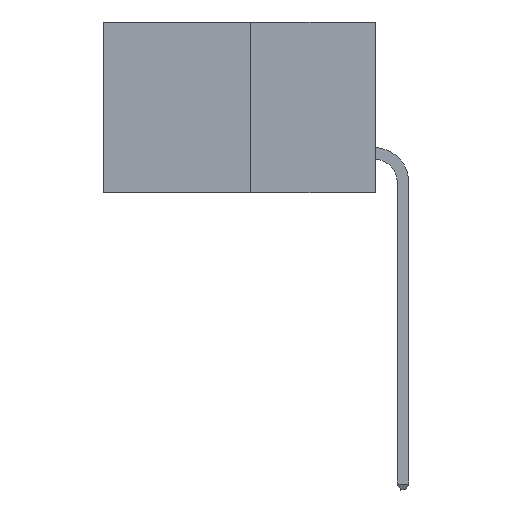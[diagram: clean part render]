
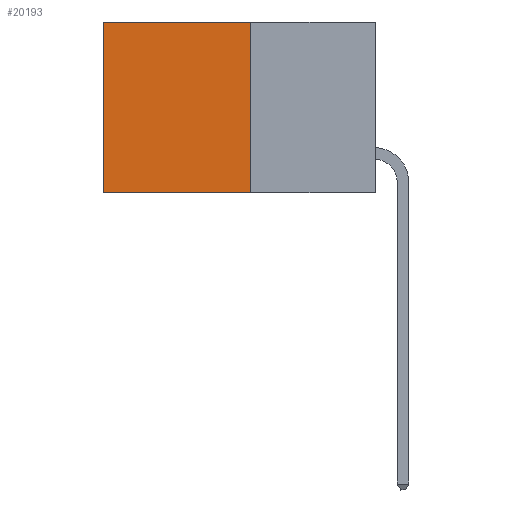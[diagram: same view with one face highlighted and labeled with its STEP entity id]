
A CAD part, left-side view. The second image highlights one B-rep face of the part: STEP entity #20193.
In plain terms, the highlighted planar face has unit normal (-1, 0, 0).
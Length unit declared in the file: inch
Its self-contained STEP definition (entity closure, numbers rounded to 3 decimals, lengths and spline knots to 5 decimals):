
#2712 = LINE ( 'NONE', #11727, #20561 ) ;
#2926 = VERTEX_POINT ( 'NONE', #3704 ) ;
#3695 = VECTOR ( 'NONE', #9438, 39.37008 ) ;
#3704 = CARTESIAN_POINT ( 'NONE',  ( 0.277, 0.59, 0. ) ) ;
#4096 = CARTESIAN_POINT ( 'NONE',  ( 0.277, 0.59, -0.37 ) ) ;
#4850 = DIRECTION ( 'NONE',  ( 0., 0., -1. ) ) ;
#5427 = DIRECTION ( 'NONE',  ( 0., 0., -1. ) ) ;
#5505 = DIRECTION ( 'NONE',  ( 1., 0., 0. ) ) ;
#6710 = AXIS2_PLACEMENT_3D ( 'NONE', #10083, #5505, #14635 ) ;
#9438 = DIRECTION ( 'NONE',  ( 0., 1., 0. ) ) ;
#9656 = ORIENTED_EDGE ( 'NONE', *, *, #17281, .T. ) ;
#10083 = CARTESIAN_POINT ( 'NONE',  ( 0.277, 0.27, -0.37 ) ) ;
#11522 = VERTEX_POINT ( 'NONE', #24267 ) ;
#11727 = CARTESIAN_POINT ( 'NONE',  ( 0.277, 0.59, -0.37 ) ) ;
#12348 = PLANE ( 'NONE',  #6710 ) ;
#14635 = DIRECTION ( 'NONE',  ( 0., 0., -1. ) ) ;
#14884 = VERTEX_POINT ( 'NONE', #4096 ) ;
#14899 = ORIENTED_EDGE ( 'NONE', *, *, #24608, .F. ) ;
#14900 = VECTOR ( 'NONE', #5427, 39.37008 ) ;
#15152 = EDGE_CURVE ( 'NONE', #11522, #2926, #15700, .T. ) ;
#15700 = LINE ( 'NONE', #25437, #21723 ) ;
#16718 = CARTESIAN_POINT ( 'NONE',  ( 0.277, 0.27, -0.37 ) ) ;
#17233 = LINE ( 'NONE', #18439, #3695 ) ;
#17281 = EDGE_CURVE ( 'NONE', #2926, #14884, #2712, .T. ) ;
#17924 = CARTESIAN_POINT ( 'NONE',  ( 0.277, 0.27, -0.37 ) ) ;
#18207 = ORIENTED_EDGE ( 'NONE', *, *, #15152, .T. ) ;
#18364 = VERTEX_POINT ( 'NONE', #17924 ) ;
#18439 = CARTESIAN_POINT ( 'NONE',  ( 0.277, 0.27, -0.37 ) ) ;
#19399 = EDGE_CURVE ( 'NONE', #18364, #14884, #17233, .T. ) ;
#20193 = ADVANCED_FACE ( 'NONE', ( #20458 ), #12348, .F. ) ;
#20211 = LINE ( 'NONE', #16718, #14900 ) ;
#20458 = FACE_OUTER_BOUND ( 'NONE', #24549, .T. ) ;
#20518 = ORIENTED_EDGE ( 'NONE', *, *, #19399, .F. ) ;
#20561 = VECTOR ( 'NONE', #4850, 39.37008 ) ;
#21723 = VECTOR ( 'NONE', #27639, 39.37008 ) ;
#24267 = CARTESIAN_POINT ( 'NONE',  ( 0.277, 0.27, 0. ) ) ;
#24549 = EDGE_LOOP ( 'NONE', ( #9656, #20518, #14899, #18207 ) ) ;
#24608 = EDGE_CURVE ( 'NONE', #11522, #18364, #20211, .T. ) ;
#25437 = CARTESIAN_POINT ( 'NONE',  ( 0.277, 0.27, 0. ) ) ;
#27639 = DIRECTION ( 'NONE',  ( 0., 1., 0. ) ) ;
